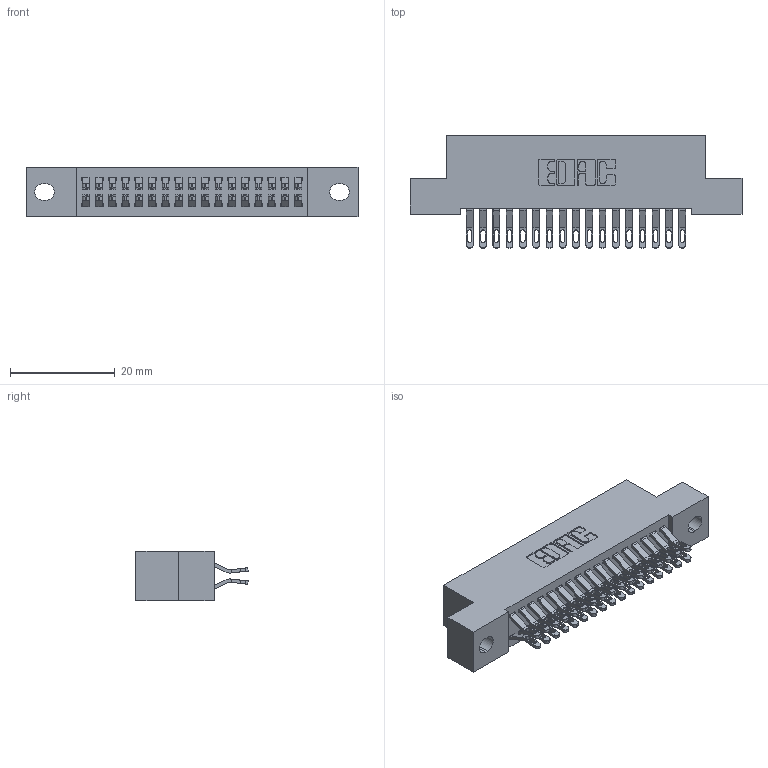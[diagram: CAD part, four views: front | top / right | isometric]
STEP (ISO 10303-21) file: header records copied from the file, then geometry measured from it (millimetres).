
FILE_DESCRIPTION (( 'STEP AP203' ), '1' );
FILE_NAME ('392-034-555-202.STEP', '2019-10-07T16:08:43', ( '' ), ( '' ), 'SwSTEP 2.0', 'SolidWorks 2016', '' );
FILE_SCHEMA (( 'CONFIG_CONTROL_DESIGN' ));
Length unit declared in the file: inch
Products named in the file (3): 342 Part_.128 Slot; 345-292-001_555 Tail; 392-034-555-202
Assembly tree (35 placements, depth 2):
  392-034-555-202
    342 Part_.128 Slot
    345-292-001_555 Tail  x34
Bounding box: 63.5 x 21.47 x 9.4 mm (x, y, z)
Volume: 5629.5 mm3; surface area: 8635.8 mm2
Topology: 35 solids, 35 shells, 2086 faces, 6533 edges, 4354 vertices
Faces by surface type: plane 1226, cylinder 860
Entity records: 14499 total; most frequent: CARTESIAN_POINT 2468, ORIENTED_EDGE 2374, DIRECTION 2123, EDGE_CURVE 1187, LINE 1039, VECTOR 1039, VERTEX_POINT 790, AXIS2_PLACEMENT_3D 542
